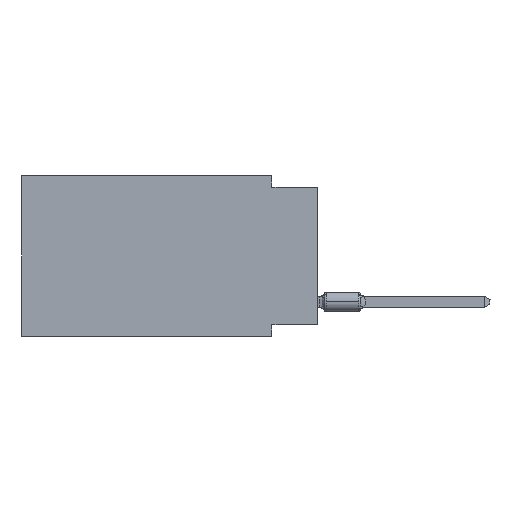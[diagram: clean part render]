
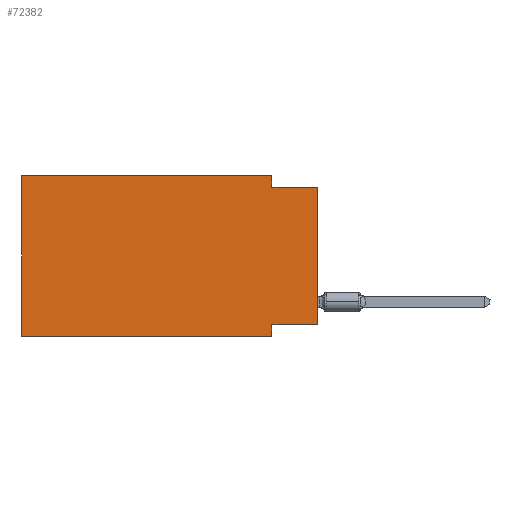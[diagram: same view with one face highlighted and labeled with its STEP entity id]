
A CAD part, left-side view. The second image highlights one B-rep face of the part: STEP entity #72382.
In plain terms, the highlighted planar face has unit normal (-1, 0, 0).
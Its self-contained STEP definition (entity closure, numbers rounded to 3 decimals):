
#509 = CARTESIAN_POINT ( 'NONE',  ( 0., 16.383, 0. ) ) ;
#1147 = DIRECTION ( 'NONE',  ( 0., 0., -1. ) ) ;
#2576 = ORIENTED_EDGE ( 'NONE', *, *, #56521, .F. ) ;
#6104 = AXIS2_PLACEMENT_3D ( 'NONE', #20030, #63808, #33515 ) ;
#12589 = VECTOR ( 'NONE', #82824, 1000. ) ;
#12721 = DIRECTION ( 'NONE',  ( 0., 0., -1. ) ) ;
#13407 = LINE ( 'NONE', #28311, #70274 ) ;
#16422 = LINE ( 'NONE', #61627, #89078 ) ;
#16513 = LINE ( 'NONE', #67513, #67725 ) ;
#19653 = CARTESIAN_POINT ( 'NONE',  ( 0., 16.383, 0. ) ) ;
#19940 = LINE ( 'NONE', #42057, #47609 ) ;
#20030 = CARTESIAN_POINT ( 'NONE',  ( 0., 16.383, 0. ) ) ;
#20754 = VERTEX_POINT ( 'NONE', #34906 ) ;
#23466 = EDGE_CURVE ( 'NONE', #20754, #88863, #13407, .T. ) ;
#25094 = VECTOR ( 'NONE', #64995, 1000. ) ;
#25701 = LINE ( 'NONE', #33388, #76569 ) ;
#26309 = FACE_OUTER_BOUND ( 'NONE', #35788, .T. ) ;
#26809 = EDGE_CURVE ( 'NONE', #48369, #83071, #19940, .T. ) ;
#27726 = PLANE ( 'NONE',  #6104 ) ;
#27822 = CARTESIAN_POINT ( 'NONE',  ( 0., 0., -0.635 ) ) ;
#28311 = CARTESIAN_POINT ( 'NONE',  ( 0., 0., -0.635 ) ) ;
#31151 = EDGE_CURVE ( 'NONE', #87992, #83071, #73141, .T. ) ;
#33388 = CARTESIAN_POINT ( 'NONE',  ( 0., 0., 0. ) ) ;
#33515 = DIRECTION ( 'NONE',  ( 0., 0., -1. ) ) ;
#34906 = CARTESIAN_POINT ( 'NONE',  ( 0., 2.54, -0.635 ) ) ;
#35706 = EDGE_CURVE ( 'NONE', #38259, #48369, #16422, .T. ) ;
#35788 = EDGE_LOOP ( 'NONE', ( #78295, #84819, #2576, #87609, #94350, #60537, #54394, #64068 ) ) ;
#38231 = EDGE_CURVE ( 'NONE', #87992, #60784, #45328, .T. ) ;
#38259 = VERTEX_POINT ( 'NONE', #45803 ) ;
#41027 = VERTEX_POINT ( 'NONE', #49623 ) ;
#42057 = CARTESIAN_POINT ( 'NONE',  ( 0., 2.54, -8.89 ) ) ;
#42862 = CARTESIAN_POINT ( 'NONE',  ( 0., 16.383, -8.89 ) ) ;
#43930 = CARTESIAN_POINT ( 'NONE',  ( 0., 2.54, -8.255 ) ) ;
#45328 = LINE ( 'NONE', #53990, #12589 ) ;
#45803 = CARTESIAN_POINT ( 'NONE',  ( 0., 0., -8.255 ) ) ;
#47609 = VECTOR ( 'NONE', #12721, 1000. ) ;
#47829 = DIRECTION ( 'NONE',  ( 0., 0., 1. ) ) ;
#48369 = VERTEX_POINT ( 'NONE', #43930 ) ;
#49623 = CARTESIAN_POINT ( 'NONE',  ( 0., 2.54, 0. ) ) ;
#52555 = CARTESIAN_POINT ( 'NONE',  ( 0., 16.383, -8.89 ) ) ;
#53990 = CARTESIAN_POINT ( 'NONE',  ( 0., 16.383, 0. ) ) ;
#54394 = ORIENTED_EDGE ( 'NONE', *, *, #26809, .F. ) ;
#56521 = EDGE_CURVE ( 'NONE', #41027, #20754, #16513, .T. ) ;
#60537 = ORIENTED_EDGE ( 'NONE', *, *, #31151, .T. ) ;
#60784 = VERTEX_POINT ( 'NONE', #19653 ) ;
#61578 = EDGE_CURVE ( 'NONE', #38259, #88863, #25701, .T. ) ;
#61627 = CARTESIAN_POINT ( 'NONE',  ( 0., 0., -8.255 ) ) ;
#63808 = DIRECTION ( 'NONE',  ( 1., 0., 0. ) ) ;
#64068 = ORIENTED_EDGE ( 'NONE', *, *, #35706, .F. ) ;
#64417 = DIRECTION ( 'NONE',  ( 0., -1., 0. ) ) ;
#64531 = DIRECTION ( 'NONE',  ( 0., -1., 0. ) ) ;
#64995 = DIRECTION ( 'NONE',  ( 0., -1., 0. ) ) ;
#67513 = CARTESIAN_POINT ( 'NONE',  ( 0., 2.54, 0. ) ) ;
#67725 = VECTOR ( 'NONE', #1147, 1000. ) ;
#70143 = EDGE_CURVE ( 'NONE', #60784, #41027, #79406, .T. ) ;
#70274 = VECTOR ( 'NONE', #64417, 1000. ) ;
#72382 = ADVANCED_FACE ( 'NONE', ( #26309 ), #27726, .F. ) ;
#73141 = LINE ( 'NONE', #42862, #25094 ) ;
#76569 = VECTOR ( 'NONE', #47829, 1000. ) ;
#78295 = ORIENTED_EDGE ( 'NONE', *, *, #61578, .T. ) ;
#79406 = LINE ( 'NONE', #509, #90399 ) ;
#82430 = CARTESIAN_POINT ( 'NONE',  ( 0., 2.54, -8.89 ) ) ;
#82824 = DIRECTION ( 'NONE',  ( 0., 0., 1. ) ) ;
#83071 = VERTEX_POINT ( 'NONE', #82430 ) ;
#84819 = ORIENTED_EDGE ( 'NONE', *, *, #23466, .F. ) ;
#87609 = ORIENTED_EDGE ( 'NONE', *, *, #70143, .F. ) ;
#87992 = VERTEX_POINT ( 'NONE', #52555 ) ;
#88863 = VERTEX_POINT ( 'NONE', #27822 ) ;
#89078 = VECTOR ( 'NONE', #90933, 1000. ) ;
#90399 = VECTOR ( 'NONE', #64531, 1000. ) ;
#90933 = DIRECTION ( 'NONE',  ( 0., 1., 0. ) ) ;
#94350 = ORIENTED_EDGE ( 'NONE', *, *, #38231, .F. ) ;
